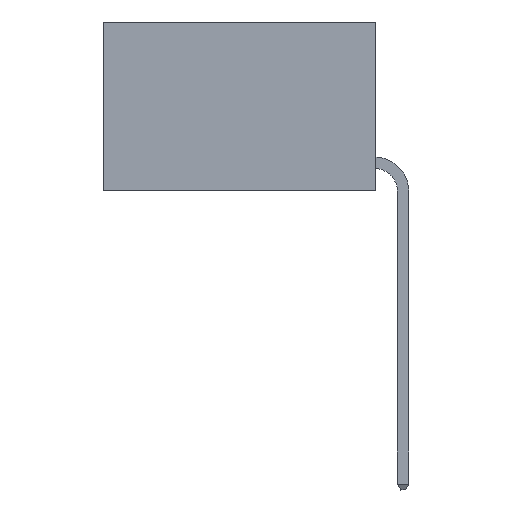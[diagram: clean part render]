
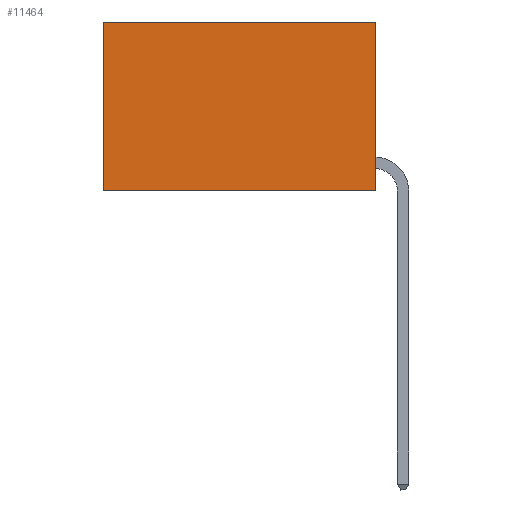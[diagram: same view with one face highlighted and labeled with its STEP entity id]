
A CAD part, left-side view. The second image highlights one B-rep face of the part: STEP entity #11464.
In plain terms, the highlighted planar face has unit normal (-1, 0, 0).
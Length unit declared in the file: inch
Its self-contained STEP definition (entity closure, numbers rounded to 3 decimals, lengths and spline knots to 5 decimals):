
#79 = FACE_OUTER_BOUND ( 'NONE', #4783, .T. ) ;
#1384 = VECTOR ( 'NONE', #10266, 39.37008 ) ;
#1446 = ORIENTED_EDGE ( 'NONE', *, *, #16950, .F. ) ;
#1717 = CARTESIAN_POINT ( 'NONE',  ( 0.2625, 0.6, -0.37 ) ) ;
#1789 = DIRECTION ( 'NONE',  ( 0., 0., -1. ) ) ;
#2032 = ORIENTED_EDGE ( 'NONE', *, *, #7631, .T. ) ;
#2291 = CARTESIAN_POINT ( 'NONE',  ( 0.2625, 0., -0.37 ) ) ;
#2376 = VERTEX_POINT ( 'NONE', #2291 ) ;
#2626 = VERTEX_POINT ( 'NONE', #1717 ) ;
#2777 = VECTOR ( 'NONE', #14743, 39.37008 ) ;
#3296 = CARTESIAN_POINT ( 'NONE',  ( 0.2625, 0., 0. ) ) ;
#3871 = DIRECTION ( 'NONE',  ( 0., 0., -1. ) ) ;
#4102 = CARTESIAN_POINT ( 'NONE',  ( 0.2625, 0.6, 0. ) ) ;
#4321 = CARTESIAN_POINT ( 'NONE',  ( 0.2625, 0., 0. ) ) ;
#4783 = EDGE_LOOP ( 'NONE', ( #2032, #1446, #15506, #12282 ) ) ;
#5496 = LINE ( 'NONE', #8780, #1384 ) ;
#6211 = DIRECTION ( 'NONE',  ( 0., 1., 0. ) ) ;
#6724 = LINE ( 'NONE', #14499, #18281 ) ;
#6887 = LINE ( 'NONE', #4102, #2777 ) ;
#6893 = EDGE_CURVE ( 'NONE', #14982, #9644, #10199, .T. ) ;
#7631 = EDGE_CURVE ( 'NONE', #9644, #2626, #6887, .T. ) ;
#8780 = CARTESIAN_POINT ( 'NONE',  ( 0.2625, 0., -0.37 ) ) ;
#9644 = VERTEX_POINT ( 'NONE', #18209 ) ;
#10199 = LINE ( 'NONE', #4321, #14210 ) ;
#10266 = DIRECTION ( 'NONE',  ( 0., 1., 0. ) ) ;
#10965 = DIRECTION ( 'NONE',  ( 1., 0., 0. ) ) ;
#11464 = ADVANCED_FACE ( 'NONE', ( #79 ), #18440, .F. ) ;
#12282 = ORIENTED_EDGE ( 'NONE', *, *, #6893, .T. ) ;
#13812 = AXIS2_PLACEMENT_3D ( 'NONE', #3296, #10965, #1789 ) ;
#13934 = EDGE_CURVE ( 'NONE', #14982, #2376, #6724, .T. ) ;
#14210 = VECTOR ( 'NONE', #6211, 39.37008 ) ;
#14499 = CARTESIAN_POINT ( 'NONE',  ( 0.2625, 0., 0. ) ) ;
#14743 = DIRECTION ( 'NONE',  ( 0., 0., -1. ) ) ;
#14982 = VERTEX_POINT ( 'NONE', #18810 ) ;
#15506 = ORIENTED_EDGE ( 'NONE', *, *, #13934, .F. ) ;
#16950 = EDGE_CURVE ( 'NONE', #2376, #2626, #5496, .T. ) ;
#18209 = CARTESIAN_POINT ( 'NONE',  ( 0.2625, 0.6, 0. ) ) ;
#18281 = VECTOR ( 'NONE', #3871, 39.37008 ) ;
#18440 = PLANE ( 'NONE',  #13812 ) ;
#18810 = CARTESIAN_POINT ( 'NONE',  ( 0.2625, 0., 0. ) ) ;
